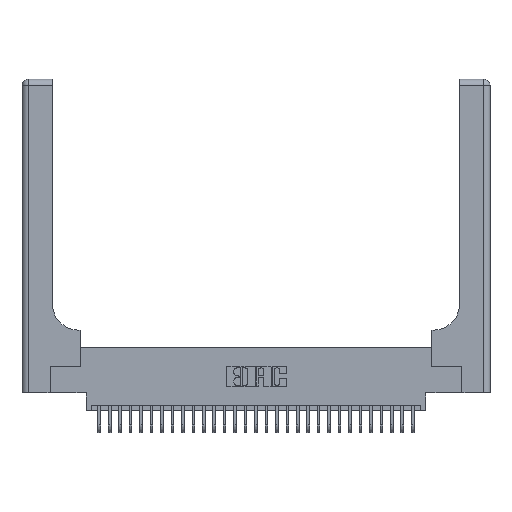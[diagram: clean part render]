
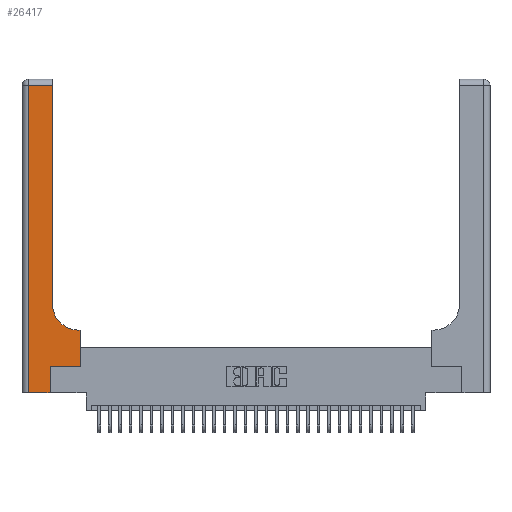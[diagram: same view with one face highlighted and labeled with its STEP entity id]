
A CAD part, top view. The second image highlights one B-rep face of the part: STEP entity #26417.
In plain terms, the highlighted planar face has unit normal (0, 0, 1).
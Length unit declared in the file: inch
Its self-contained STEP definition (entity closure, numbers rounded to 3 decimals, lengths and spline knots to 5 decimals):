
#553 = ORIENTED_EDGE ( 'NONE', *, *, #25131, .T. ) ;
#589 = CARTESIAN_POINT ( 'NONE',  ( 0.5585, 0.25, 0.37 ) ) ;
#1257 = DIRECTION ( 'NONE',  ( -1., 0., 0. ) ) ;
#2162 = ORIENTED_EDGE ( 'NONE', *, *, #27308, .T. ) ;
#2412 = EDGE_CURVE ( 'NONE', #10685, #12239, #24535, .T. ) ;
#2734 = AXIS2_PLACEMENT_3D ( 'NONE', #6667, #9293, #26997 ) ;
#3005 = CARTESIAN_POINT ( 'NONE',  ( 0.269, 0., 0.37 ) ) ;
#3165 = DIRECTION ( 'NONE',  ( 0., 1., 0. ) ) ;
#3349 = ORIENTED_EDGE ( 'NONE', *, *, #7625, .T. ) ;
#4061 = VECTOR ( 'NONE', #10581, 39.37008 ) ;
#4146 = EDGE_CURVE ( 'NONE', #19265, #23376, #28828, .T. ) ;
#4230 = VERTEX_POINT ( 'NONE', #26272 ) ;
#4240 = VECTOR ( 'NONE', #1257, 39.37008 ) ;
#4849 = VERTEX_POINT ( 'NONE', #3005 ) ;
#4956 = VECTOR ( 'NONE', #10259, 39.37008 ) ;
#5159 = DIRECTION ( 'NONE',  ( 0., 1., 0. ) ) ;
#6667 = CARTESIAN_POINT ( 'NONE',  ( 0., 3., 0.37 ) ) ;
#6946 = VERTEX_POINT ( 'NONE', #32343 ) ;
#7625 = EDGE_CURVE ( 'NONE', #12239, #4230, #17416, .T. ) ;
#7778 = VERTEX_POINT ( 'NONE', #10156 ) ;
#7816 = CARTESIAN_POINT ( 'NONE',  ( 0.5585, 0.6, 0.37 ) ) ;
#8589 = ORIENTED_EDGE ( 'NONE', *, *, #4146, .T. ) ;
#8609 = VECTOR ( 'NONE', #3165, 39.37008 ) ;
#9293 = DIRECTION ( 'NONE',  ( 0., 0., -1. ) ) ;
#10156 = CARTESIAN_POINT ( 'NONE',  ( 0.2915, 0.85, 0.37 ) ) ;
#10259 = DIRECTION ( 'NONE',  ( 0., 1., 0. ) ) ;
#10581 = DIRECTION ( 'NONE',  ( -1., 0., 0. ) ) ;
#10685 = VERTEX_POINT ( 'NONE', #12269 ) ;
#11094 = FACE_OUTER_BOUND ( 'NONE', #28473, .T. ) ;
#11150 = CIRCLE ( 'NONE', #25081, 0.25 ) ;
#11472 = VECTOR ( 'NONE', #12291, 39.37008 ) ;
#12239 = VERTEX_POINT ( 'NONE', #26876 ) ;
#12269 = CARTESIAN_POINT ( 'NONE',  ( 0.2915, 2.94, 0.37 ) ) ;
#12291 = DIRECTION ( 'NONE',  ( 0., -1., 0. ) ) ;
#12315 = DIRECTION ( 'NONE',  ( 0., 0., -1. ) ) ;
#12620 = LINE ( 'NONE', #30463, #4956 ) ;
#12627 = VECTOR ( 'NONE', #23947, 39.37008 ) ;
#13441 = LINE ( 'NONE', #28830, #12627 ) ;
#14063 = EDGE_CURVE ( 'NONE', #6946, #7778, #11150, .T. ) ;
#15739 = CARTESIAN_POINT ( 'NONE',  ( 0.269, 0.25, 0.37 ) ) ;
#16459 = CARTESIAN_POINT ( 'NONE',  ( 0.5585, 0.25, 0.37 ) ) ;
#16982 = ORIENTED_EDGE ( 'NONE', *, *, #14063, .T. ) ;
#17327 = EDGE_CURVE ( 'NONE', #23376, #6946, #24355, .T. ) ;
#17416 = LINE ( 'NONE', #27407, #11472 ) ;
#17541 = CARTESIAN_POINT ( 'NONE',  ( 0., 0., 0.37 ) ) ;
#19265 = VERTEX_POINT ( 'NONE', #16459 ) ;
#20460 = CARTESIAN_POINT ( 'NONE',  ( 0.2915, 3., 0.37 ) ) ;
#20481 = EDGE_CURVE ( 'NONE', #31406, #19265, #13441, .T. ) ;
#21922 = PLANE ( 'NONE',  #2734 ) ;
#22058 = ORIENTED_EDGE ( 'NONE', *, *, #22196, .T. ) ;
#22087 = ORIENTED_EDGE ( 'NONE', *, *, #17327, .T. ) ;
#22196 = EDGE_CURVE ( 'NONE', #7778, #10685, #29521, .T. ) ;
#22242 = LINE ( 'NONE', #17541, #28955 ) ;
#22814 = VECTOR ( 'NONE', #5159, 39.37008 ) ;
#22844 = ORIENTED_EDGE ( 'NONE', *, *, #2412, .T. ) ;
#23376 = VERTEX_POINT ( 'NONE', #7816 ) ;
#23947 = DIRECTION ( 'NONE',  ( 1., 0., 0. ) ) ;
#24355 = LINE ( 'NONE', #30765, #4061 ) ;
#24535 = LINE ( 'NONE', #31620, #4240 ) ;
#25081 = AXIS2_PLACEMENT_3D ( 'NONE', #27424, #12315, #29947 ) ;
#25131 = EDGE_CURVE ( 'NONE', #4230, #4849, #22242, .T. ) ;
#26272 = CARTESIAN_POINT ( 'NONE',  ( 0.06, 0., 0.37 ) ) ;
#26417 = ADVANCED_FACE ( 'NONE', ( #11094 ), #21922, .F. ) ;
#26876 = CARTESIAN_POINT ( 'NONE',  ( 0.06, 2.94, 0.37 ) ) ;
#26997 = DIRECTION ( 'NONE',  ( -1., 0., 0. ) ) ;
#27308 = EDGE_CURVE ( 'NONE', #4849, #31406, #12620, .T. ) ;
#27407 = CARTESIAN_POINT ( 'NONE',  ( 0.06, 3., 0.37 ) ) ;
#27424 = CARTESIAN_POINT ( 'NONE',  ( 0.5415, 0.85, 0.37 ) ) ;
#28473 = EDGE_LOOP ( 'NONE', ( #22058, #22844, #3349, #553, #2162, #30736, #8589, #22087, #16982 ) ) ;
#28828 = LINE ( 'NONE', #589, #8609 ) ;
#28830 = CARTESIAN_POINT ( 'NONE',  ( 0.269, 0.25, 0.37 ) ) ;
#28955 = VECTOR ( 'NONE', #32549, 39.37008 ) ;
#29521 = LINE ( 'NONE', #20460, #22814 ) ;
#29947 = DIRECTION ( 'NONE',  ( 1., 0., 0. ) ) ;
#30463 = CARTESIAN_POINT ( 'NONE',  ( 0.269, 0., 0.37 ) ) ;
#30736 = ORIENTED_EDGE ( 'NONE', *, *, #20481, .T. ) ;
#30765 = CARTESIAN_POINT ( 'NONE',  ( 0.2915, 0.6, 0.37 ) ) ;
#31406 = VERTEX_POINT ( 'NONE', #15739 ) ;
#31620 = CARTESIAN_POINT ( 'NONE',  ( 0., 2.94, 0.37 ) ) ;
#32343 = CARTESIAN_POINT ( 'NONE',  ( 0.5415, 0.6, 0.37 ) ) ;
#32549 = DIRECTION ( 'NONE',  ( 1., 0., 0. ) ) ;
